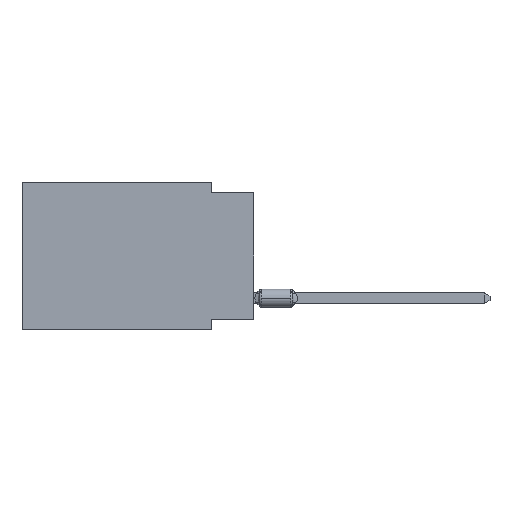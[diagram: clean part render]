
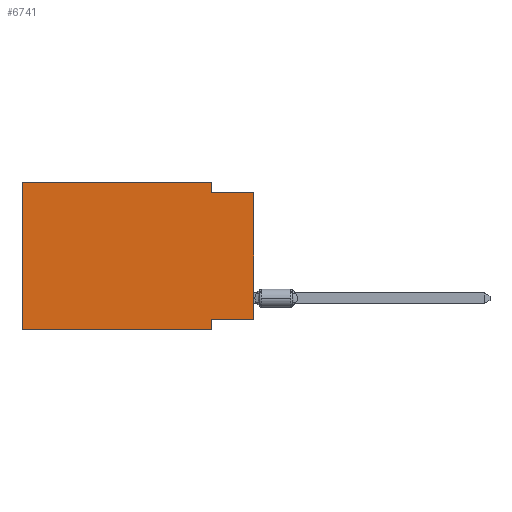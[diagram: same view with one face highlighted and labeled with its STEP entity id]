
A CAD part, left-side view. The second image highlights one B-rep face of the part: STEP entity #6741.
In plain terms, the highlighted planar face has unit normal (-1, 0, 0).
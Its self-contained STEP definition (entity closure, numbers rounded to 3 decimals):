
#107 = AXIS2_PLACEMENT_3D ( 'NONE', #1213, #2280, #2121 ) ;
#188 = EDGE_CURVE ( 'NONE', #11565, #8123, #9238, .T. ) ;
#408 = ORIENTED_EDGE ( 'NONE', *, *, #446, .F. ) ;
#414 = CARTESIAN_POINT ( 'NONE',  ( 0., 0., -8.255 ) ) ;
#446 = EDGE_CURVE ( 'NONE', #11760, #5617, #12315, .T. ) ;
#605 = CARTESIAN_POINT ( 'NONE',  ( 0., 2.54, -8.89 ) ) ;
#710 = EDGE_CURVE ( 'NONE', #5617, #9636, #13263, .T. ) ;
#749 = CARTESIAN_POINT ( 'NONE',  ( 0., 13.97, 0. ) ) ;
#1213 = CARTESIAN_POINT ( 'NONE',  ( 0., 13.97, 0. ) ) ;
#1295 = CARTESIAN_POINT ( 'NONE',  ( 0., 0., 0. ) ) ;
#1305 = VECTOR ( 'NONE', #13275, 1000. ) ;
#1350 = LINE ( 'NONE', #1420, #8006 ) ;
#1420 = CARTESIAN_POINT ( 'NONE',  ( 0., 13.97, -8.89 ) ) ;
#1914 = CARTESIAN_POINT ( 'NONE',  ( 0., 2.54, 0. ) ) ;
#2068 = CARTESIAN_POINT ( 'NONE',  ( 0., 2.54, -8.89 ) ) ;
#2121 = DIRECTION ( 'NONE',  ( 0., 0., -1. ) ) ;
#2280 = DIRECTION ( 'NONE',  ( 1., 0., 0. ) ) ;
#2446 = DIRECTION ( 'NONE',  ( 0., 1., 0. ) ) ;
#2464 = VERTEX_POINT ( 'NONE', #10321 ) ;
#2692 = CARTESIAN_POINT ( 'NONE',  ( 0., 2.54, -0.635 ) ) ;
#3431 = CARTESIAN_POINT ( 'NONE',  ( 0., 2.54, -8.255 ) ) ;
#3478 = PLANE ( 'NONE',  #107 ) ;
#3577 = EDGE_LOOP ( 'NONE', ( #8757, #8287, #408, #3965, #4348, #13078, #12006, #8996 ) ) ;
#3819 = VERTEX_POINT ( 'NONE', #6692 ) ;
#3965 = ORIENTED_EDGE ( 'NONE', *, *, #10930, .F. ) ;
#4348 = ORIENTED_EDGE ( 'NONE', *, *, #7092, .F. ) ;
#4533 = DIRECTION ( 'NONE',  ( 0., 0., 1. ) ) ;
#4685 = EDGE_CURVE ( 'NONE', #11565, #9636, #13090, .T. ) ;
#5617 = VERTEX_POINT ( 'NONE', #2692 ) ;
#5675 = EDGE_CURVE ( 'NONE', #8123, #9609, #13506, .T. ) ;
#6163 = CARTESIAN_POINT ( 'NONE',  ( 0., 0., -0.635 ) ) ;
#6651 = LINE ( 'NONE', #749, #13801 ) ;
#6692 = CARTESIAN_POINT ( 'NONE',  ( 0., 13.97, 0. ) ) ;
#6741 = ADVANCED_FACE ( 'NONE', ( #6968 ), #3478, .F. ) ;
#6873 = LINE ( 'NONE', #11256, #13174 ) ;
#6968 = FACE_OUTER_BOUND ( 'NONE', #3577, .T. ) ;
#7092 = EDGE_CURVE ( 'NONE', #2464, #3819, #6873, .T. ) ;
#8006 = VECTOR ( 'NONE', #9502, 1000. ) ;
#8123 = VERTEX_POINT ( 'NONE', #3431 ) ;
#8287 = ORIENTED_EDGE ( 'NONE', *, *, #710, .F. ) ;
#8757 = ORIENTED_EDGE ( 'NONE', *, *, #4685, .T. ) ;
#8906 = VECTOR ( 'NONE', #12037, 1000. ) ;
#8988 = DIRECTION ( 'NONE',  ( 0., -1., 0. ) ) ;
#8996 = ORIENTED_EDGE ( 'NONE', *, *, #188, .F. ) ;
#9238 = LINE ( 'NONE', #12787, #12479 ) ;
#9502 = DIRECTION ( 'NONE',  ( 0., -1., 0. ) ) ;
#9522 = DIRECTION ( 'NONE',  ( 0., 0., 1. ) ) ;
#9609 = VERTEX_POINT ( 'NONE', #605 ) ;
#9636 = VERTEX_POINT ( 'NONE', #10735 ) ;
#9720 = VECTOR ( 'NONE', #9522, 1000. ) ;
#10321 = CARTESIAN_POINT ( 'NONE',  ( 0., 13.97, -8.89 ) ) ;
#10735 = CARTESIAN_POINT ( 'NONE',  ( 0., 0., -0.635 ) ) ;
#10930 = EDGE_CURVE ( 'NONE', #3819, #11760, #6651, .T. ) ;
#11256 = CARTESIAN_POINT ( 'NONE',  ( 0., 13.97, 0. ) ) ;
#11306 = EDGE_CURVE ( 'NONE', #2464, #9609, #1350, .T. ) ;
#11565 = VERTEX_POINT ( 'NONE', #414 ) ;
#11760 = VERTEX_POINT ( 'NONE', #1914 ) ;
#12006 = ORIENTED_EDGE ( 'NONE', *, *, #5675, .F. ) ;
#12037 = DIRECTION ( 'NONE',  ( 0., -1., 0. ) ) ;
#12315 = LINE ( 'NONE', #14532, #13512 ) ;
#12479 = VECTOR ( 'NONE', #2446, 1000. ) ;
#12787 = CARTESIAN_POINT ( 'NONE',  ( 0., 0., -8.255 ) ) ;
#13078 = ORIENTED_EDGE ( 'NONE', *, *, #11306, .T. ) ;
#13090 = LINE ( 'NONE', #1295, #9720 ) ;
#13174 = VECTOR ( 'NONE', #4533, 1000. ) ;
#13263 = LINE ( 'NONE', #6163, #8906 ) ;
#13275 = DIRECTION ( 'NONE',  ( 0., 0., -1. ) ) ;
#13506 = LINE ( 'NONE', #2068, #1305 ) ;
#13512 = VECTOR ( 'NONE', #14608, 1000. ) ;
#13801 = VECTOR ( 'NONE', #8988, 1000. ) ;
#14532 = CARTESIAN_POINT ( 'NONE',  ( 0., 2.54, 0. ) ) ;
#14608 = DIRECTION ( 'NONE',  ( 0., 0., -1. ) ) ;
